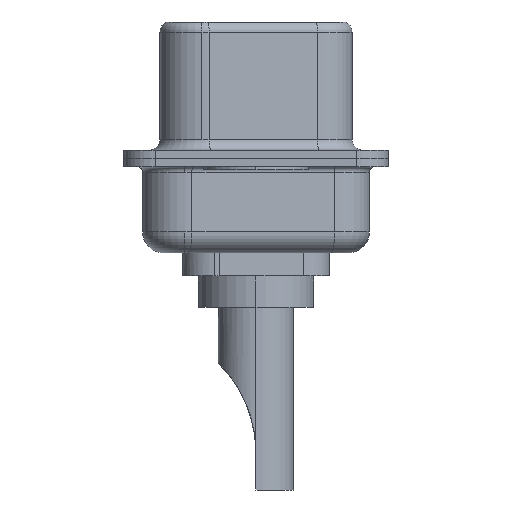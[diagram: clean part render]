
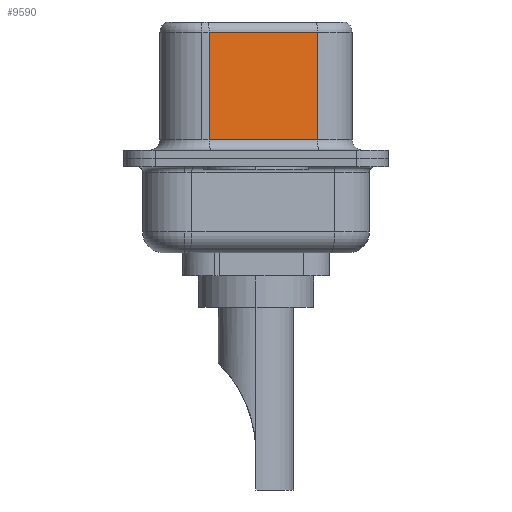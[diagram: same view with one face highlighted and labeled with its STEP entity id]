
A CAD part, left-side view. The second image highlights one B-rep face of the part: STEP entity #9590.
In plain terms, the highlighted planar face has unit normal (-0.985, -0.174, 0).
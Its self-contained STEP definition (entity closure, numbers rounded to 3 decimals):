
#58 = VECTOR ( 'NONE', #6857, 1000. ) ;
#222 = DIRECTION ( 'NONE',  ( 0., 0., -1. ) ) ;
#299 = LINE ( 'NONE', #7588, #11375 ) ;
#391 = ORIENTED_EDGE ( 'NONE', *, *, #2431, .T. ) ;
#434 = LINE ( 'NONE', #7223, #58 ) ;
#577 = VERTEX_POINT ( 'NONE', #13392 ) ;
#634 = CARTESIAN_POINT ( 'NONE',  ( 4.565, -2.927, 6.52 ) ) ;
#653 = LINE ( 'NONE', #1134, #12056 ) ;
#745 = VERTEX_POINT ( 'NONE', #5639 ) ;
#1134 = CARTESIAN_POINT ( 'NONE',  ( 4.565, -2.927, 6.52 ) ) ;
#1739 = DIRECTION ( 'NONE',  ( -0.174, 0.985, 0. ) ) ;
#2369 = EDGE_CURVE ( 'NONE', #745, #577, #653, .T. ) ;
#2431 = EDGE_CURVE ( 'NONE', #6168, #8937, #299, .T. ) ;
#2512 = FACE_OUTER_BOUND ( 'NONE', #11596, .T. ) ;
#2794 = AXIS2_PLACEMENT_3D ( 'NONE', #634, #8410, #1739 ) ;
#4055 = DIRECTION ( 'NONE',  ( 0., 0., -1. ) ) ;
#4758 = EDGE_CURVE ( 'NONE', #8937, #577, #434, .T. ) ;
#5464 = CARTESIAN_POINT ( 'NONE',  ( 4.565, -2.927, 6.02 ) ) ;
#5639 = CARTESIAN_POINT ( 'NONE',  ( 4.565, -2.927, 6.02 ) ) ;
#6168 = VERTEX_POINT ( 'NONE', #13647 ) ;
#6470 = DIRECTION ( 'NONE',  ( -0.174, 0.985, 0. ) ) ;
#6625 = EDGE_CURVE ( 'NONE', #745, #6168, #13053, .T. ) ;
#6857 = DIRECTION ( 'NONE',  ( 0.174, -0.985, 0. ) ) ;
#7223 = CARTESIAN_POINT ( 'NONE',  ( 4.565, -2.927, 0.9 ) ) ;
#7588 = CARTESIAN_POINT ( 'NONE',  ( 3.655, 2.233, 6.52 ) ) ;
#8344 = ORIENTED_EDGE ( 'NONE', *, *, #4758, .T. ) ;
#8364 = PLANE ( 'NONE',  #2794 ) ;
#8410 = DIRECTION ( 'NONE',  ( 0.985, 0.174, 0. ) ) ;
#8937 = VERTEX_POINT ( 'NONE', #10406 ) ;
#9443 = ORIENTED_EDGE ( 'NONE', *, *, #6625, .T. ) ;
#9590 = ADVANCED_FACE ( 'NONE', ( #2512 ), #8364, .F. ) ;
#10406 = CARTESIAN_POINT ( 'NONE',  ( 3.655, 2.233, 0.9 ) ) ;
#11375 = VECTOR ( 'NONE', #222, 1000. ) ;
#11596 = EDGE_LOOP ( 'NONE', ( #13050, #9443, #391, #8344 ) ) ;
#12056 = VECTOR ( 'NONE', #4055, 1000. ) ;
#12726 = VECTOR ( 'NONE', #6470, 1000. ) ;
#13050 = ORIENTED_EDGE ( 'NONE', *, *, #2369, .F. ) ;
#13053 = LINE ( 'NONE', #5464, #12726 ) ;
#13392 = CARTESIAN_POINT ( 'NONE',  ( 4.565, -2.927, 0.9 ) ) ;
#13647 = CARTESIAN_POINT ( 'NONE',  ( 3.655, 2.233, 6.02 ) ) ;
